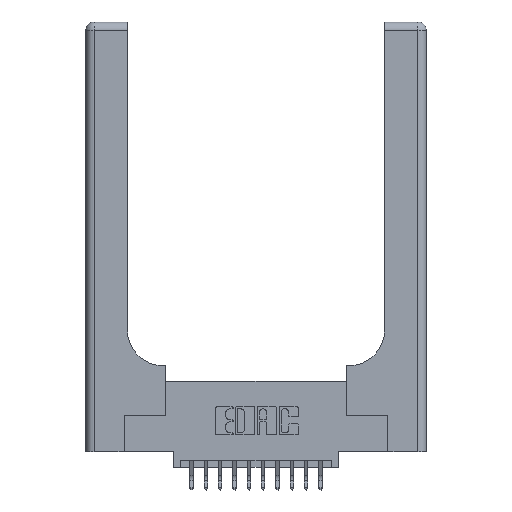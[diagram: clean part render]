
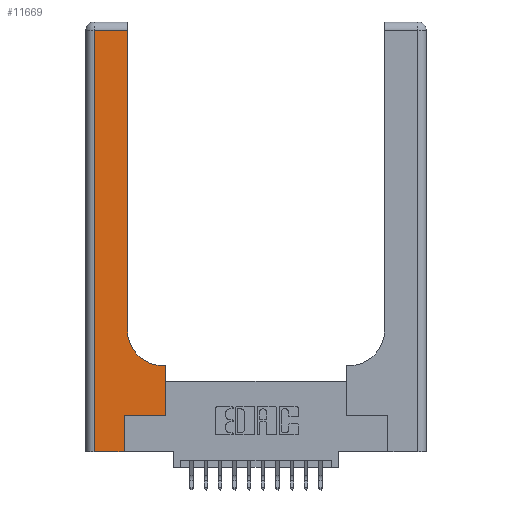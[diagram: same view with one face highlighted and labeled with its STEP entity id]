
A CAD part, top view. The second image highlights one B-rep face of the part: STEP entity #11669.
In plain terms, the highlighted planar face has unit normal (0, 0, 1).
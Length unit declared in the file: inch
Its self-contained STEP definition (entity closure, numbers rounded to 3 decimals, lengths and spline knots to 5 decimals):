
#39 = EDGE_CURVE ( 'NONE', #8463, #5532, #11244, .T. ) ;
#49 = CARTESIAN_POINT ( 'NONE',  ( 0.2915, 2.94, 0.37 ) ) ;
#413 = VERTEX_POINT ( 'NONE', #49 ) ;
#621 = CARTESIAN_POINT ( 'NONE',  ( 0., 0., 0.37 ) ) ;
#701 = ORIENTED_EDGE ( 'NONE', *, *, #39, .T. ) ;
#1153 = EDGE_CURVE ( 'NONE', #16535, #8463, #2849, .T. ) ;
#1658 = CARTESIAN_POINT ( 'NONE',  ( 0.06, 2.94, 0.37 ) ) ;
#2277 = ORIENTED_EDGE ( 'NONE', *, *, #5715, .T. ) ;
#2381 = LINE ( 'NONE', #14139, #15918 ) ;
#2689 = EDGE_LOOP ( 'NONE', ( #12656, #2277, #6372, #13494, #10814, #14360, #4039, #11235, #701 ) ) ;
#2758 = DIRECTION ( 'NONE',  ( 0., 1., 0. ) ) ;
#2849 = LINE ( 'NONE', #11002, #10517 ) ;
#2941 = EDGE_CURVE ( 'NONE', #13138, #14533, #2381, .T. ) ;
#3165 = VERTEX_POINT ( 'NONE', #4511 ) ;
#3182 = DIRECTION ( 'NONE',  ( -1., 0., 0. ) ) ;
#3436 = CARTESIAN_POINT ( 'NONE',  ( 0.269, 0., 0.37 ) ) ;
#3500 = VECTOR ( 'NONE', #6243, 39.37008 ) ;
#4039 = ORIENTED_EDGE ( 'NONE', *, *, #5955, .T. ) ;
#4215 = CARTESIAN_POINT ( 'NONE',  ( 0.06, 0., 0.37 ) ) ;
#4511 = CARTESIAN_POINT ( 'NONE',  ( 0.5585, 0.25, 0.37 ) ) ;
#4583 = AXIS2_PLACEMENT_3D ( 'NONE', #6834, #16214, #8202 ) ;
#5058 = CARTESIAN_POINT ( 'NONE',  ( 0.269, 0.25, 0.37 ) ) ;
#5109 = CARTESIAN_POINT ( 'NONE',  ( 0.5585, 0.25, 0.37 ) ) ;
#5315 = VECTOR ( 'NONE', #2758, 39.37008 ) ;
#5532 = VERTEX_POINT ( 'NONE', #14932 ) ;
#5715 = EDGE_CURVE ( 'NONE', #413, #13138, #5760, .T. ) ;
#5760 = LINE ( 'NONE', #9948, #12456 ) ;
#5955 = EDGE_CURVE ( 'NONE', #3165, #16535, #9544, .T. ) ;
#6243 = DIRECTION ( 'NONE',  ( 1., 0., 0. ) ) ;
#6372 = ORIENTED_EDGE ( 'NONE', *, *, #2941, .T. ) ;
#6399 = CARTESIAN_POINT ( 'NONE',  ( 0.269, 0.25, 0.37 ) ) ;
#6834 = CARTESIAN_POINT ( 'NONE',  ( 0., 3., 0.37 ) ) ;
#7714 = DIRECTION ( 'NONE',  ( 0., 1., 0. ) ) ;
#7782 = DIRECTION ( 'NONE',  ( 1., 0., 0. ) ) ;
#7833 = DIRECTION ( 'NONE',  ( 0., 1., 0. ) ) ;
#8202 = DIRECTION ( 'NONE',  ( -1., 0., 0. ) ) ;
#8281 = VECTOR ( 'NONE', #7782, 39.37008 ) ;
#8331 = EDGE_CURVE ( 'NONE', #14533, #13872, #14259, .T. ) ;
#8463 = VERTEX_POINT ( 'NONE', #14517 ) ;
#9335 = FACE_OUTER_BOUND ( 'NONE', #2689, .T. ) ;
#9429 = DIRECTION ( 'NONE',  ( 1., 0., 0. ) ) ;
#9544 = LINE ( 'NONE', #5109, #12659 ) ;
#9764 = DIRECTION ( 'NONE',  ( 0., 0., -1. ) ) ;
#9769 = CARTESIAN_POINT ( 'NONE',  ( 0.5415, 0.85, 0.37 ) ) ;
#9948 = CARTESIAN_POINT ( 'NONE',  ( 0., 2.94, 0.37 ) ) ;
#10405 = CARTESIAN_POINT ( 'NONE',  ( 0.269, 0., 0.37 ) ) ;
#10517 = VECTOR ( 'NONE', #10982, 39.37008 ) ;
#10814 = ORIENTED_EDGE ( 'NONE', *, *, #15838, .T. ) ;
#10982 = DIRECTION ( 'NONE',  ( -1., 0., 0. ) ) ;
#11002 = CARTESIAN_POINT ( 'NONE',  ( 0.2915, 0.6, 0.37 ) ) ;
#11235 = ORIENTED_EDGE ( 'NONE', *, *, #1153, .T. ) ;
#11244 = CIRCLE ( 'NONE', #14686, 0.25 ) ;
#11669 = ADVANCED_FACE ( 'NONE', ( #9335 ), #14874, .F. ) ;
#11678 = EDGE_CURVE ( 'NONE', #5532, #413, #16451, .T. ) ;
#12226 = LINE ( 'NONE', #6399, #8281 ) ;
#12456 = VECTOR ( 'NONE', #3182, 39.37008 ) ;
#12656 = ORIENTED_EDGE ( 'NONE', *, *, #11678, .T. ) ;
#12659 = VECTOR ( 'NONE', #7833, 39.37008 ) ;
#12688 = VERTEX_POINT ( 'NONE', #5058 ) ;
#12690 = EDGE_CURVE ( 'NONE', #12688, #3165, #12226, .T. ) ;
#12829 = DIRECTION ( 'NONE',  ( 0., -1., 0. ) ) ;
#13138 = VERTEX_POINT ( 'NONE', #1658 ) ;
#13272 = CARTESIAN_POINT ( 'NONE',  ( 0.5585, 0.6, 0.37 ) ) ;
#13494 = ORIENTED_EDGE ( 'NONE', *, *, #8331, .T. ) ;
#13500 = CARTESIAN_POINT ( 'NONE',  ( 0.2915, 3., 0.37 ) ) ;
#13675 = VECTOR ( 'NONE', #7714, 39.37008 ) ;
#13872 = VERTEX_POINT ( 'NONE', #3436 ) ;
#14139 = CARTESIAN_POINT ( 'NONE',  ( 0.06, 3., 0.37 ) ) ;
#14259 = LINE ( 'NONE', #621, #3500 ) ;
#14360 = ORIENTED_EDGE ( 'NONE', *, *, #12690, .T. ) ;
#14517 = CARTESIAN_POINT ( 'NONE',  ( 0.5415, 0.6, 0.37 ) ) ;
#14533 = VERTEX_POINT ( 'NONE', #4215 ) ;
#14686 = AXIS2_PLACEMENT_3D ( 'NONE', #9769, #9764, #9429 ) ;
#14874 = PLANE ( 'NONE',  #4583 ) ;
#14932 = CARTESIAN_POINT ( 'NONE',  ( 0.2915, 0.85, 0.37 ) ) ;
#15838 = EDGE_CURVE ( 'NONE', #13872, #12688, #17269, .T. ) ;
#15918 = VECTOR ( 'NONE', #12829, 39.37008 ) ;
#16214 = DIRECTION ( 'NONE',  ( 0., 0., -1. ) ) ;
#16451 = LINE ( 'NONE', #13500, #5315 ) ;
#16535 = VERTEX_POINT ( 'NONE', #13272 ) ;
#17269 = LINE ( 'NONE', #10405, #13675 ) ;
